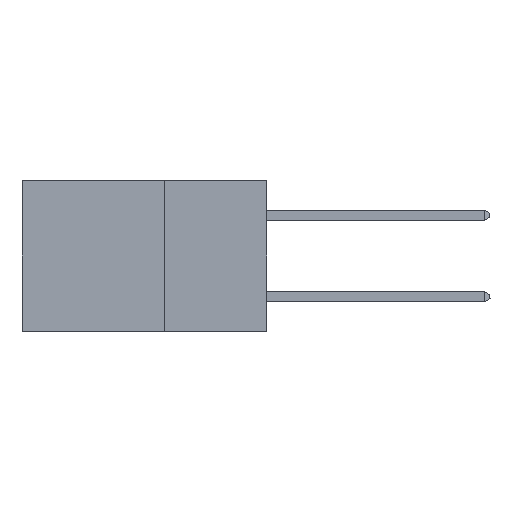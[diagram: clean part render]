
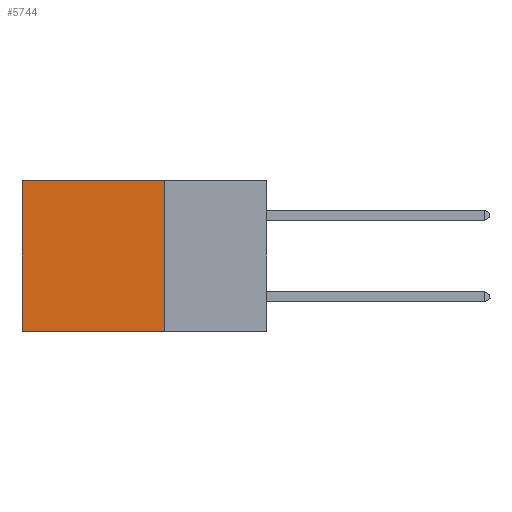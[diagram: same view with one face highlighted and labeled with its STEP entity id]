
A CAD part, left-side view. The second image highlights one B-rep face of the part: STEP entity #5744.
In plain terms, the highlighted planar face has unit normal (-1, 0, 0).
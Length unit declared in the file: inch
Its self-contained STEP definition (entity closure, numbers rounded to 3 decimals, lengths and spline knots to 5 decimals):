
#169 = ORIENTED_EDGE ( 'NONE', *, *, #8708, .T. ) ;
#286 = EDGE_CURVE ( 'NONE', #12359, #4209, #7949, .T. ) ;
#421 = CARTESIAN_POINT ( 'NONE',  ( 0.2875, 0.25, 0. ) ) ;
#2044 = CARTESIAN_POINT ( 'NONE',  ( 0.2875, 0.25, 0. ) ) ;
#2244 = DIRECTION ( 'NONE',  ( 1., 0., 0. ) ) ;
#2529 = LINE ( 'NONE', #11213, #9730 ) ;
#2535 = CARTESIAN_POINT ( 'NONE',  ( 0.2875, 0.6, -0.37 ) ) ;
#2604 = FACE_OUTER_BOUND ( 'NONE', #4148, .T. ) ;
#3727 = DIRECTION ( 'NONE',  ( 0., 0., -1. ) ) ;
#4052 = DIRECTION ( 'NONE',  ( 0., 0., -1. ) ) ;
#4148 = EDGE_LOOP ( 'NONE', ( #169, #12657, #15270, #6212 ) ) ;
#4209 = VERTEX_POINT ( 'NONE', #10039 ) ;
#4253 = VERTEX_POINT ( 'NONE', #12809 ) ;
#4666 = VERTEX_POINT ( 'NONE', #2535 ) ;
#5744 = ADVANCED_FACE ( 'NONE', ( #2604 ), #6546, .F. ) ;
#6212 = ORIENTED_EDGE ( 'NONE', *, *, #15396, .T. ) ;
#6546 = PLANE ( 'NONE',  #13554 ) ;
#7022 = DIRECTION ( 'NONE',  ( 0., 1., 0. ) ) ;
#7333 = LINE ( 'NONE', #2044, #14402 ) ;
#7645 = CARTESIAN_POINT ( 'NONE',  ( 0.2875, 0.25, 0. ) ) ;
#7949 = LINE ( 'NONE', #421, #11257 ) ;
#8708 = EDGE_CURVE ( 'NONE', #4253, #4666, #2529, .T. ) ;
#9730 = VECTOR ( 'NONE', #4052, 39.37008 ) ;
#9880 = VECTOR ( 'NONE', #7022, 39.37008 ) ;
#10039 = CARTESIAN_POINT ( 'NONE',  ( 0.2875, 0.25, -0.37 ) ) ;
#10643 = EDGE_CURVE ( 'NONE', #4209, #4666, #16925, .T. ) ;
#10850 = CARTESIAN_POINT ( 'NONE',  ( 0.2875, 0.25, 0. ) ) ;
#11213 = CARTESIAN_POINT ( 'NONE',  ( 0.2875, 0.6, 0. ) ) ;
#11257 = VECTOR ( 'NONE', #3727, 39.37008 ) ;
#12277 = DIRECTION ( 'NONE',  ( 0., 0., -1. ) ) ;
#12359 = VERTEX_POINT ( 'NONE', #7645 ) ;
#12657 = ORIENTED_EDGE ( 'NONE', *, *, #10643, .F. ) ;
#12809 = CARTESIAN_POINT ( 'NONE',  ( 0.2875, 0.6, 0. ) ) ;
#13554 = AXIS2_PLACEMENT_3D ( 'NONE', #10850, #2244, #12277 ) ;
#14402 = VECTOR ( 'NONE', #17693, 39.37008 ) ;
#15270 = ORIENTED_EDGE ( 'NONE', *, *, #286, .F. ) ;
#15396 = EDGE_CURVE ( 'NONE', #12359, #4253, #7333, .T. ) ;
#16917 = CARTESIAN_POINT ( 'NONE',  ( 0.2875, 0.25, -0.37 ) ) ;
#16925 = LINE ( 'NONE', #16917, #9880 ) ;
#17693 = DIRECTION ( 'NONE',  ( 0., 1., 0. ) ) ;
